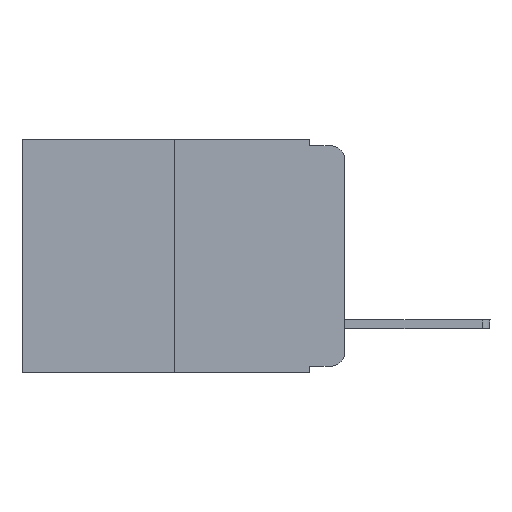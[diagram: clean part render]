
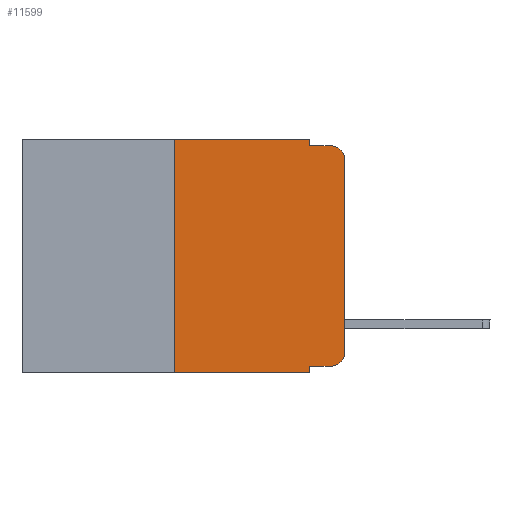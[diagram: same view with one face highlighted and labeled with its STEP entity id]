
A CAD part, left-side view. The second image highlights one B-rep face of the part: STEP entity #11599.
In plain terms, the highlighted planar face has unit normal (-1, 0, 0).
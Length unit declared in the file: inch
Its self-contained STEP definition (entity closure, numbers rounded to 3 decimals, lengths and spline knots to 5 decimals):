
#221 = LINE ( 'NONE', #11539, #1828 ) ;
#661 = AXIS2_PLACEMENT_3D ( 'NONE', #7869, #11235, #11307 ) ;
#840 = VECTOR ( 'NONE', #13848, 39.37008 ) ;
#1097 = EDGE_CURVE ( 'NONE', #3890, #3531, #10082, .T. ) ;
#1719 = CARTESIAN_POINT ( 'NONE',  ( 0., 0.02, -0.01 ) ) ;
#1828 = VECTOR ( 'NONE', #3505, 39.37008 ) ;
#1873 = LINE ( 'NONE', #6323, #11608 ) ;
#1880 = ORIENTED_EDGE ( 'NONE', *, *, #13989, .F. ) ;
#2012 = LINE ( 'NONE', #12103, #4589 ) ;
#2093 = DIRECTION ( 'NONE',  ( 1., 0., 0. ) ) ;
#2146 = CARTESIAN_POINT ( 'NONE',  ( 0., 0.02, -0.333 ) ) ;
#2569 = EDGE_CURVE ( 'NONE', #6656, #7477, #12668, .T. ) ;
#2693 = VECTOR ( 'NONE', #11646, 39.37008 ) ;
#2707 = VECTOR ( 'NONE', #13125, 39.37008 ) ;
#2754 = CIRCLE ( 'NONE', #661, 0.02 ) ;
#3010 = ORIENTED_EDGE ( 'NONE', *, *, #3378, .F. ) ;
#3041 = DIRECTION ( 'NONE',  ( 0., 0., -1. ) ) ;
#3049 = CARTESIAN_POINT ( 'NONE',  ( 0., 0., 0. ) ) ;
#3254 = EDGE_LOOP ( 'NONE', ( #10958, #8839, #3010, #7183, #11091, #11527, #14325, #1880, #5782, #6920 ) ) ;
#3378 = EDGE_CURVE ( 'NONE', #10142, #5870, #221, .T. ) ;
#3457 = CARTESIAN_POINT ( 'NONE',  ( 0., 0.25, 0. ) ) ;
#3505 = DIRECTION ( 'NONE',  ( 0., -1., 0. ) ) ;
#3511 = VERTEX_POINT ( 'NONE', #7287 ) ;
#3531 = VERTEX_POINT ( 'NONE', #7218 ) ;
#3790 = CARTESIAN_POINT ( 'NONE',  ( 0., 0.02, -0.03 ) ) ;
#3890 = VERTEX_POINT ( 'NONE', #9374 ) ;
#4349 = DIRECTION ( 'NONE',  ( 0., -1., 0. ) ) ;
#4589 = VECTOR ( 'NONE', #6468, 39.37008 ) ;
#5074 = VERTEX_POINT ( 'NONE', #7992 ) ;
#5350 = VERTEX_POINT ( 'NONE', #2146 ) ;
#5754 = EDGE_CURVE ( 'NONE', #5350, #7459, #2754, .T. ) ;
#5782 = ORIENTED_EDGE ( 'NONE', *, *, #11584, .T. ) ;
#5870 = VERTEX_POINT ( 'NONE', #1719 ) ;
#6055 = LINE ( 'NONE', #9470, #840 ) ;
#6202 = CARTESIAN_POINT ( 'NONE',  ( 0., 0.051, 0. ) ) ;
#6323 = CARTESIAN_POINT ( 'NONE',  ( 0., 0.051, 0. ) ) ;
#6468 = DIRECTION ( 'NONE',  ( 0., -1., 0. ) ) ;
#6656 = VERTEX_POINT ( 'NONE', #3457 ) ;
#6920 = ORIENTED_EDGE ( 'NONE', *, *, #5754, .T. ) ;
#6929 = DIRECTION ( 'NONE',  ( 0., 0., -1. ) ) ;
#7004 = DIRECTION ( 'NONE',  ( -1., 0., 0. ) ) ;
#7183 = ORIENTED_EDGE ( 'NONE', *, *, #7334, .F. ) ;
#7218 = CARTESIAN_POINT ( 'NONE',  ( 0., 0.051, -0.343 ) ) ;
#7287 = CARTESIAN_POINT ( 'NONE',  ( 0., 0., -0.03 ) ) ;
#7334 = EDGE_CURVE ( 'NONE', #7477, #10142, #13861, .T. ) ;
#7459 = VERTEX_POINT ( 'NONE', #10795 ) ;
#7477 = VERTEX_POINT ( 'NONE', #11684 ) ;
#7869 = CARTESIAN_POINT ( 'NONE',  ( 0., 0.02, -0.313 ) ) ;
#7992 = CARTESIAN_POINT ( 'NONE',  ( 0., 0.051, -0.333 ) ) ;
#8551 = CIRCLE ( 'NONE', #10894, 0.02 ) ;
#8707 = CARTESIAN_POINT ( 'NONE',  ( 0., 0.473, -0.343 ) ) ;
#8782 = FACE_OUTER_BOUND ( 'NONE', #3254, .T. ) ;
#8839 = ORIENTED_EDGE ( 'NONE', *, *, #12349, .T. ) ;
#9374 = CARTESIAN_POINT ( 'NONE',  ( 0., 0.25, -0.343 ) ) ;
#9470 = CARTESIAN_POINT ( 'NONE',  ( 0., 0.25, 0. ) ) ;
#9478 = AXIS2_PLACEMENT_3D ( 'NONE', #9874, #2093, #9808 ) ;
#9808 = DIRECTION ( 'NONE',  ( 0., 0., -1. ) ) ;
#9874 = CARTESIAN_POINT ( 'NONE',  ( 0., 0.473, 0. ) ) ;
#9888 = VECTOR ( 'NONE', #4349, 39.37008 ) ;
#10082 = LINE ( 'NONE', #8707, #9888 ) ;
#10142 = VERTEX_POINT ( 'NONE', #12306 ) ;
#10722 = DIRECTION ( 'NONE',  ( 0., 0., -1. ) ) ;
#10778 = LINE ( 'NONE', #3049, #2707 ) ;
#10795 = CARTESIAN_POINT ( 'NONE',  ( 0., 0., -0.313 ) ) ;
#10894 = AXIS2_PLACEMENT_3D ( 'NONE', #3790, #7004, #6929 ) ;
#10958 = ORIENTED_EDGE ( 'NONE', *, *, #11200, .T. ) ;
#11091 = ORIENTED_EDGE ( 'NONE', *, *, #2569, .F. ) ;
#11116 = EDGE_CURVE ( 'NONE', #3890, #6656, #6055, .T. ) ;
#11200 = EDGE_CURVE ( 'NONE', #7459, #3511, #10778, .T. ) ;
#11235 = DIRECTION ( 'NONE',  ( -1., 0., 0. ) ) ;
#11307 = DIRECTION ( 'NONE',  ( 0., 0., -1. ) ) ;
#11527 = ORIENTED_EDGE ( 'NONE', *, *, #11116, .F. ) ;
#11539 = CARTESIAN_POINT ( 'NONE',  ( 0., 0.051, -0.01 ) ) ;
#11584 = EDGE_CURVE ( 'NONE', #5074, #5350, #2012, .T. ) ;
#11599 = ADVANCED_FACE ( 'NONE', ( #8782 ), #14410, .F. ) ;
#11608 = VECTOR ( 'NONE', #3041, 39.37008 ) ;
#11646 = DIRECTION ( 'NONE',  ( 0., -1., 0. ) ) ;
#11684 = CARTESIAN_POINT ( 'NONE',  ( 0., 0.051, 0. ) ) ;
#12103 = CARTESIAN_POINT ( 'NONE',  ( 0., 0.051, -0.333 ) ) ;
#12306 = CARTESIAN_POINT ( 'NONE',  ( 0., 0.051, -0.01 ) ) ;
#12349 = EDGE_CURVE ( 'NONE', #3511, #5870, #8551, .T. ) ;
#12668 = LINE ( 'NONE', #13614, #2693 ) ;
#13125 = DIRECTION ( 'NONE',  ( 0., 0., 1. ) ) ;
#13614 = CARTESIAN_POINT ( 'NONE',  ( 0., 0.473, 0. ) ) ;
#13848 = DIRECTION ( 'NONE',  ( 0., 0., 1. ) ) ;
#13861 = LINE ( 'NONE', #6202, #13871 ) ;
#13871 = VECTOR ( 'NONE', #10722, 39.37008 ) ;
#13989 = EDGE_CURVE ( 'NONE', #5074, #3531, #1873, .T. ) ;
#14325 = ORIENTED_EDGE ( 'NONE', *, *, #1097, .T. ) ;
#14410 = PLANE ( 'NONE',  #9478 ) ;
